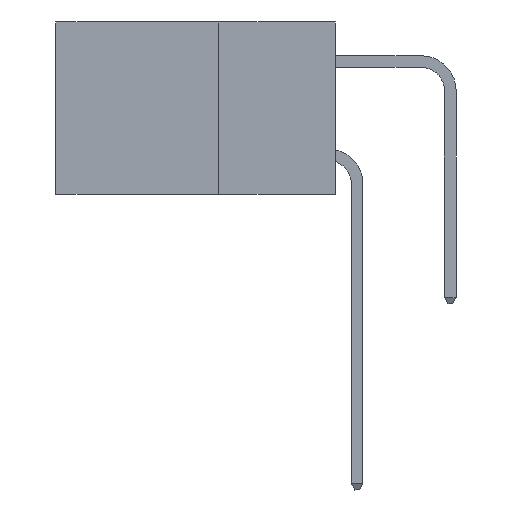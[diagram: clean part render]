
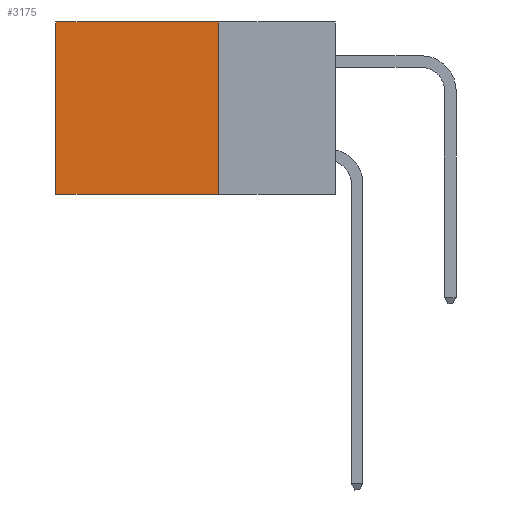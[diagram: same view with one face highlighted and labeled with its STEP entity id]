
A CAD part, left-side view. The second image highlights one B-rep face of the part: STEP entity #3175.
In plain terms, the highlighted planar face has unit normal (-1, 0, 0).
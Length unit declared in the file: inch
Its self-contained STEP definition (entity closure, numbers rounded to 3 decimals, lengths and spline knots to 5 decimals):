
#101 = DIRECTION ( 'NONE',  ( 0., 1., 0. ) ) ;
#1857 = CARTESIAN_POINT ( 'NONE',  ( 0.2875, 0.25, 0. ) ) ;
#2587 = CARTESIAN_POINT ( 'NONE',  ( 0.2875, 0.25, 0. ) ) ;
#2750 = VECTOR ( 'NONE', #101, 39.37008 ) ;
#3175 = ADVANCED_FACE ( 'NONE', ( #7293 ), #25217, .F. ) ;
#4464 = AXIS2_PLACEMENT_3D ( 'NONE', #23311, #13798, #20923 ) ;
#4564 = LINE ( 'NONE', #7623, #13902 ) ;
#5550 = ORIENTED_EDGE ( 'NONE', *, *, #7731, .F. ) ;
#7293 = FACE_OUTER_BOUND ( 'NONE', #29622, .T. ) ;
#7623 = CARTESIAN_POINT ( 'NONE',  ( 0.2875, 0.6, 0. ) ) ;
#7731 = EDGE_CURVE ( 'NONE', #26518, #8323, #24285, .T. ) ;
#7876 = EDGE_CURVE ( 'NONE', #20359, #8323, #4564, .T. ) ;
#8323 = VERTEX_POINT ( 'NONE', #10635 ) ;
#9096 = DIRECTION ( 'NONE',  ( 0., 1., 0. ) ) ;
#9706 = DIRECTION ( 'NONE',  ( 0., 0., -1. ) ) ;
#10635 = CARTESIAN_POINT ( 'NONE',  ( 0.2875, 0.6, -0.37 ) ) ;
#12288 = CARTESIAN_POINT ( 'NONE',  ( 0.2875, 0.6, 0. ) ) ;
#13798 = DIRECTION ( 'NONE',  ( 1., 0., 0. ) ) ;
#13902 = VECTOR ( 'NONE', #9706, 39.37008 ) ;
#16297 = VERTEX_POINT ( 'NONE', #26157 ) ;
#17113 = DIRECTION ( 'NONE',  ( 0., 0., -1. ) ) ;
#17278 = VECTOR ( 'NONE', #17113, 39.37008 ) ;
#18275 = ORIENTED_EDGE ( 'NONE', *, *, #7876, .T. ) ;
#18620 = LINE ( 'NONE', #1857, #24187 ) ;
#20359 = VERTEX_POINT ( 'NONE', #12288 ) ;
#20471 = CARTESIAN_POINT ( 'NONE',  ( 0.2875, 0.25, -0.37 ) ) ;
#20675 = ORIENTED_EDGE ( 'NONE', *, *, #23303, .T. ) ;
#20923 = DIRECTION ( 'NONE',  ( 0., 0., -1. ) ) ;
#23303 = EDGE_CURVE ( 'NONE', #16297, #20359, #18620, .T. ) ;
#23311 = CARTESIAN_POINT ( 'NONE',  ( 0.2875, 0.25, 0. ) ) ;
#24002 = EDGE_CURVE ( 'NONE', #16297, #26518, #25105, .T. ) ;
#24187 = VECTOR ( 'NONE', #9096, 39.37008 ) ;
#24285 = LINE ( 'NONE', #28447, #2750 ) ;
#25105 = LINE ( 'NONE', #2587, #17278 ) ;
#25217 = PLANE ( 'NONE',  #4464 ) ;
#26157 = CARTESIAN_POINT ( 'NONE',  ( 0.2875, 0.25, 0. ) ) ;
#26518 = VERTEX_POINT ( 'NONE', #20471 ) ;
#26548 = ORIENTED_EDGE ( 'NONE', *, *, #24002, .F. ) ;
#28447 = CARTESIAN_POINT ( 'NONE',  ( 0.2875, 0.25, -0.37 ) ) ;
#29622 = EDGE_LOOP ( 'NONE', ( #18275, #5550, #26548, #20675 ) ) ;
